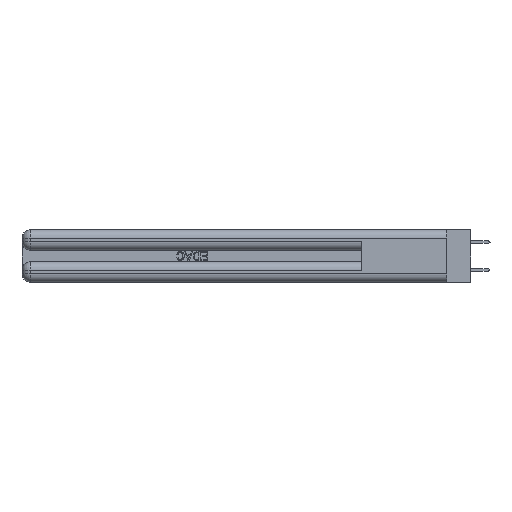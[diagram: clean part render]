
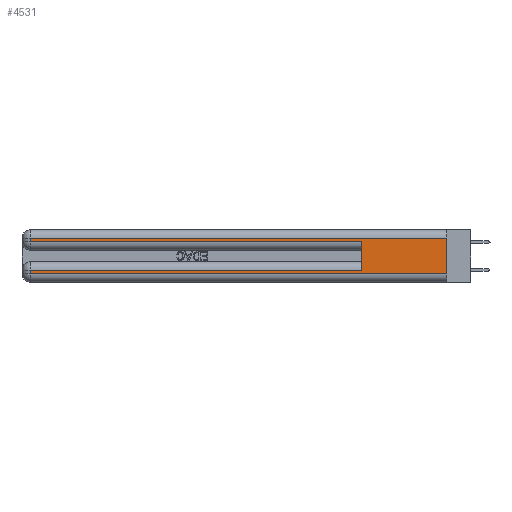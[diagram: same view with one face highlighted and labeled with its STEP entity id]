
A CAD part, left-side view. The second image highlights one B-rep face of the part: STEP entity #4531.
In plain terms, the highlighted planar face has unit normal (-1, 0, 0).
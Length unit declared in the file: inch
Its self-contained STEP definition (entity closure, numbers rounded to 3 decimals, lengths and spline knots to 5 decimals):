
#869 = LINE ( 'NONE', #28608, #5127 ) ;
#1313 = CARTESIAN_POINT ( 'NONE',  ( 0., 0., 0.37 ) ) ;
#2670 = LINE ( 'NONE', #41204, #13382 ) ;
#2814 = DIRECTION ( 'NONE',  ( 0., 0., -1. ) ) ;
#4531 = ADVANCED_FACE ( 'NONE', ( #41351 ), #37234, .F. ) ;
#4564 = ORIENTED_EDGE ( 'NONE', *, *, #40676, .T. ) ;
#4695 = EDGE_CURVE ( 'NONE', #9864, #25987, #18011, .T. ) ;
#4870 = DIRECTION ( 'NONE',  ( 0., 1., 0. ) ) ;
#5127 = VECTOR ( 'NONE', #31450, 39.37008 ) ;
#5281 = AXIS2_PLACEMENT_3D ( 'NONE', #1313, #21116, #17022 ) ;
#5626 = EDGE_CURVE ( 'NONE', #24583, #41436, #41972, .T. ) ;
#5899 = EDGE_CURVE ( 'NONE', #48763, #25987, #32380, .T. ) ;
#5918 = CARTESIAN_POINT ( 'NONE',  ( 0., 2.94, 0.085 ) ) ;
#9864 = VERTEX_POINT ( 'NONE', #12702 ) ;
#10952 = CARTESIAN_POINT ( 'NONE',  ( 0., 0.6, 0.085 ) ) ;
#12702 = CARTESIAN_POINT ( 'NONE',  ( 0., 0., 0.31 ) ) ;
#12751 = VECTOR ( 'NONE', #4870, 39.37008 ) ;
#12785 = VERTEX_POINT ( 'NONE', #18772 ) ;
#13382 = VECTOR ( 'NONE', #34013, 39.37008 ) ;
#14287 = VERTEX_POINT ( 'NONE', #5918 ) ;
#14637 = CARTESIAN_POINT ( 'NONE',  ( 0., 0., 0.285 ) ) ;
#16738 = EDGE_CURVE ( 'NONE', #14287, #48763, #869, .T. ) ;
#17022 = DIRECTION ( 'NONE',  ( 0., 0., -1. ) ) ;
#17858 = EDGE_CURVE ( 'NONE', #24804, #12785, #49431, .T. ) ;
#18011 = LINE ( 'NONE', #29782, #29030 ) ;
#18484 = LINE ( 'NONE', #14637, #47645 ) ;
#18772 = CARTESIAN_POINT ( 'NONE',  ( 0., 2.94, 0.285 ) ) ;
#20831 = ORIENTED_EDGE ( 'NONE', *, *, #23187, .T. ) ;
#21116 = DIRECTION ( 'NONE',  ( 1., 0., 0. ) ) ;
#21986 = DIRECTION ( 'NONE',  ( 0., 0., 1. ) ) ;
#22238 = CARTESIAN_POINT ( 'NONE',  ( 0., 0.6, 0.285 ) ) ;
#23187 = EDGE_CURVE ( 'NONE', #9864, #24804, #2670, .T. ) ;
#24583 = VERTEX_POINT ( 'NONE', #10952 ) ;
#24804 = VERTEX_POINT ( 'NONE', #35342 ) ;
#25177 = CARTESIAN_POINT ( 'NONE',  ( 0., 2.94, 0.06 ) ) ;
#25842 = ORIENTED_EDGE ( 'NONE', *, *, #4695, .F. ) ;
#25987 = VERTEX_POINT ( 'NONE', #49397 ) ;
#27227 = EDGE_LOOP ( 'NONE', ( #25842, #20831, #35738, #36369, #43867, #4564, #39888, #31772 ) ) ;
#28217 = LINE ( 'NONE', #40028, #12751 ) ;
#28608 = CARTESIAN_POINT ( 'NONE',  ( 0., 2.94, 0.37 ) ) ;
#29030 = VECTOR ( 'NONE', #2814, 39.37008 ) ;
#29661 = CARTESIAN_POINT ( 'NONE',  ( 0., 0.6, 0.145 ) ) ;
#29782 = CARTESIAN_POINT ( 'NONE',  ( 0., 0., 0.37 ) ) ;
#30258 = DIRECTION ( 'NONE',  ( 0., -1., 0. ) ) ;
#31450 = DIRECTION ( 'NONE',  ( 0., 0., -1. ) ) ;
#31772 = ORIENTED_EDGE ( 'NONE', *, *, #5899, .T. ) ;
#31999 = VECTOR ( 'NONE', #37876, 39.37008 ) ;
#32380 = LINE ( 'NONE', #43911, #36503 ) ;
#32445 = EDGE_CURVE ( 'NONE', #12785, #41436, #18484, .T. ) ;
#34013 = DIRECTION ( 'NONE',  ( 0., 1., 0. ) ) ;
#35342 = CARTESIAN_POINT ( 'NONE',  ( 0., 2.94, 0.31 ) ) ;
#35738 = ORIENTED_EDGE ( 'NONE', *, *, #17858, .T. ) ;
#36369 = ORIENTED_EDGE ( 'NONE', *, *, #32445, .T. ) ;
#36468 = DIRECTION ( 'NONE',  ( 0., -1., 0. ) ) ;
#36503 = VECTOR ( 'NONE', #36468, 39.37008 ) ;
#37234 = PLANE ( 'NONE',  #5281 ) ;
#37876 = DIRECTION ( 'NONE',  ( 0., 0., -1. ) ) ;
#39888 = ORIENTED_EDGE ( 'NONE', *, *, #16738, .T. ) ;
#40028 = CARTESIAN_POINT ( 'NONE',  ( 0., 0., 0.085 ) ) ;
#40676 = EDGE_CURVE ( 'NONE', #24583, #14287, #28217, .T. ) ;
#41204 = CARTESIAN_POINT ( 'NONE',  ( 0., 0., 0.31 ) ) ;
#41351 = FACE_OUTER_BOUND ( 'NONE', #27227, .T. ) ;
#41436 = VERTEX_POINT ( 'NONE', #22238 ) ;
#41972 = LINE ( 'NONE', #29661, #45499 ) ;
#43867 = ORIENTED_EDGE ( 'NONE', *, *, #5626, .F. ) ;
#43911 = CARTESIAN_POINT ( 'NONE',  ( 0., 0., 0.06 ) ) ;
#44811 = CARTESIAN_POINT ( 'NONE',  ( 0., 2.94, 0.37 ) ) ;
#45499 = VECTOR ( 'NONE', #21986, 39.37008 ) ;
#47645 = VECTOR ( 'NONE', #30258, 39.37008 ) ;
#48763 = VERTEX_POINT ( 'NONE', #25177 ) ;
#49397 = CARTESIAN_POINT ( 'NONE',  ( 0., 0., 0.06 ) ) ;
#49431 = LINE ( 'NONE', #44811, #31999 ) ;
